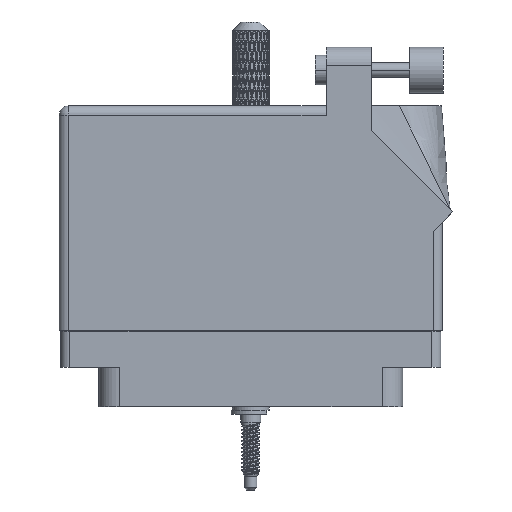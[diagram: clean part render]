
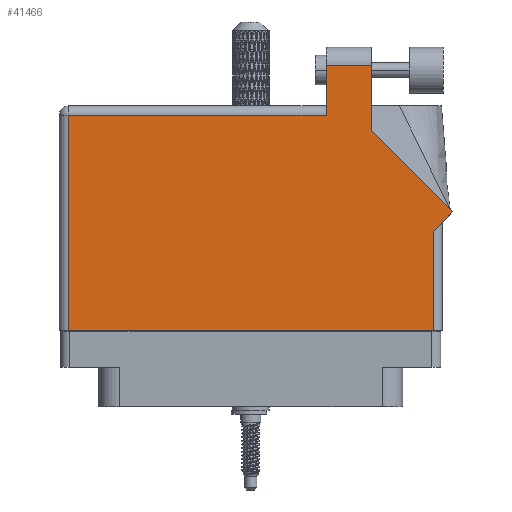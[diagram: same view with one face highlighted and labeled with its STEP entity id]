
A CAD part, front view. The second image highlights one B-rep face of the part: STEP entity #41466.
In plain terms, the highlighted face is planar.
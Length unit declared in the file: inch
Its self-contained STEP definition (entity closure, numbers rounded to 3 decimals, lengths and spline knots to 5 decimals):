
#833 = LINE ( 'NONE', #73050, #27924 ) ;
#3703 = DIRECTION ( 'NONE',  ( -0.707, 0.707, 0. ) ) ;
#4800 = CARTESIAN_POINT ( 'NONE',  ( 1.37671, 0.70771, 0.455 ) ) ;
#9196 = ORIENTED_EDGE ( 'NONE', *, *, #9268, .T. ) ;
#9268 = EDGE_CURVE ( 'NONE', #10494, #92738, #107664, .T. ) ;
#10494 = VERTEX_POINT ( 'NONE', #89354 ) ;
#14965 = ORIENTED_EDGE ( 'NONE', *, *, #43762, .T. ) ;
#16027 = CARTESIAN_POINT ( 'NONE',  ( 0.82, 1.26442, 0.455 ) ) ;
#18230 = AXIS2_PLACEMENT_3D ( 'NONE', #114415, #78236, #87043 ) ;
#18638 = VECTOR ( 'NONE', #3703, 39.37008 ) ;
#19224 = LINE ( 'NONE', #42667, #20700 ) ;
#20197 = ORIENTED_EDGE ( 'NONE', *, *, #50325, .T. ) ;
#20525 = ORIENTED_EDGE ( 'NONE', *, *, #61420, .T. ) ;
#20700 = VECTOR ( 'NONE', #32016, 39.37008 ) ;
#21903 = ORIENTED_EDGE ( 'NONE', *, *, #105423, .T. ) ;
#22416 = FACE_OUTER_BOUND ( 'NONE', #34664, .T. ) ;
#23545 = PLANE ( 'NONE',  #18230 ) ;
#26065 = DIRECTION ( 'NONE',  ( 0.707, 0.707, 0. ) ) ;
#27645 = CARTESIAN_POINT ( 'NONE',  ( 0.513, 1.705, 0.455 ) ) ;
#27924 = VECTOR ( 'NONE', #90976, 39.37008 ) ;
#30039 = CARTESIAN_POINT ( 'NONE',  ( 0.82, 1.705, 0.455 ) ) ;
#30421 = CARTESIAN_POINT ( 'NONE',  ( 1.244, -0.1, 0.455 ) ) ;
#32016 = DIRECTION ( 'NONE',  ( -1., 0., 0. ) ) ;
#34664 = EDGE_LOOP ( 'NONE', ( #88670, #46800, #20525, #14965, #20197, #9196, #21903, #92643, #40899 ) ) ;
#36629 = EDGE_CURVE ( 'NONE', #66441, #113163, #59986, .T. ) ;
#36643 = EDGE_CURVE ( 'NONE', #95723, #66441, #41450, .T. ) ;
#38893 = LINE ( 'NONE', #60615, #95616 ) ;
#40820 = DIRECTION ( 'NONE',  ( 0., -1., 0. ) ) ;
#40899 = ORIENTED_EDGE ( 'NONE', *, *, #36643, .T. ) ;
#41450 = LINE ( 'NONE', #100964, #18638 ) ;
#41466 = ADVANCED_FACE ( 'NONE', ( #22416 ), #23545, .F. ) ;
#42007 = DIRECTION ( 'NONE',  ( 0., -1., 0. ) ) ;
#42667 = CARTESIAN_POINT ( 'NONE',  ( -1.306, 1.368, 0.455 ) ) ;
#43382 = VECTOR ( 'NONE', #60351, 39.37008 ) ;
#43762 = EDGE_CURVE ( 'NONE', #115823, #106742, #19224, .T. ) ;
#45214 = DIRECTION ( 'NONE',  ( 1., 0., 0. ) ) ;
#45949 = CARTESIAN_POINT ( 'NONE',  ( 0.513, 1.368, 0.455 ) ) ;
#46800 = ORIENTED_EDGE ( 'NONE', *, *, #77039, .T. ) ;
#49828 = DIRECTION ( 'NONE',  ( 0., 1., 0. ) ) ;
#50325 = EDGE_CURVE ( 'NONE', #106742, #10494, #38893, .T. ) ;
#59986 = LINE ( 'NONE', #111629, #67100 ) ;
#60351 = DIRECTION ( 'NONE',  ( 0., 1., 0. ) ) ;
#60615 = CARTESIAN_POINT ( 'NONE',  ( -1.244, -0.1, 0.455 ) ) ;
#61420 = EDGE_CURVE ( 'NONE', #77894, #115823, #72012, .T. ) ;
#62138 = CARTESIAN_POINT ( 'NONE',  ( 1.306, 0.637, 0.455 ) ) ;
#62706 = VECTOR ( 'NONE', #26065, 39.37008 ) ;
#66441 = VERTEX_POINT ( 'NONE', #16027 ) ;
#67100 = VECTOR ( 'NONE', #49828, 39.37008 ) ;
#72012 = LINE ( 'NONE', #96298, #106134 ) ;
#73050 = CARTESIAN_POINT ( 'NONE',  ( 0.513, 1.705, 0.455 ) ) ;
#74837 = CARTESIAN_POINT ( 'NONE',  ( 1.244, 0.575, 0.455 ) ) ;
#77039 = EDGE_CURVE ( 'NONE', #113163, #77894, #833, .T. ) ;
#77894 = VERTEX_POINT ( 'NONE', #27645 ) ;
#78236 = DIRECTION ( 'NONE',  ( 0., 0., -1. ) ) ;
#81360 = EDGE_CURVE ( 'NONE', #103806, #95723, #86860, .T. ) ;
#86860 = LINE ( 'NONE', #62138, #62706 ) ;
#87043 = DIRECTION ( 'NONE',  ( -1., 0., 0. ) ) ;
#88505 = CARTESIAN_POINT ( 'NONE',  ( 1.244, 0.637, 0.455 ) ) ;
#88670 = ORIENTED_EDGE ( 'NONE', *, *, #36629, .T. ) ;
#89354 = CARTESIAN_POINT ( 'NONE',  ( -1.244, -0.1, 0.455 ) ) ;
#90976 = DIRECTION ( 'NONE',  ( -1., 0., 0. ) ) ;
#91579 = LINE ( 'NONE', #88505, #43382 ) ;
#92643 = ORIENTED_EDGE ( 'NONE', *, *, #81360, .T. ) ;
#92738 = VERTEX_POINT ( 'NONE', #30421 ) ;
#95616 = VECTOR ( 'NONE', #40820, 39.37008 ) ;
#95723 = VERTEX_POINT ( 'NONE', #4800 ) ;
#96298 = CARTESIAN_POINT ( 'NONE',  ( 0.513, 1.43, 0.455 ) ) ;
#99487 = CARTESIAN_POINT ( 'NONE',  ( -1.306, -0.1, 0.455 ) ) ;
#100964 = CARTESIAN_POINT ( 'NONE',  ( 1.37671, 0.70771, 0.455 ) ) ;
#103806 = VERTEX_POINT ( 'NONE', #74837 ) ;
#104093 = CARTESIAN_POINT ( 'NONE',  ( -1.244, 1.368, 0.455 ) ) ;
#104839 = VECTOR ( 'NONE', #45214, 39.37008 ) ;
#105423 = EDGE_CURVE ( 'NONE', #92738, #103806, #91579, .T. ) ;
#106134 = VECTOR ( 'NONE', #42007, 39.37008 ) ;
#106742 = VERTEX_POINT ( 'NONE', #104093 ) ;
#107664 = LINE ( 'NONE', #99487, #104839 ) ;
#111629 = CARTESIAN_POINT ( 'NONE',  ( 0.82, 1.26442, 0.455 ) ) ;
#113163 = VERTEX_POINT ( 'NONE', #30039 ) ;
#114415 = CARTESIAN_POINT ( 'NONE',  ( -1.306, 1.43, 0.455 ) ) ;
#115823 = VERTEX_POINT ( 'NONE', #45949 ) ;
